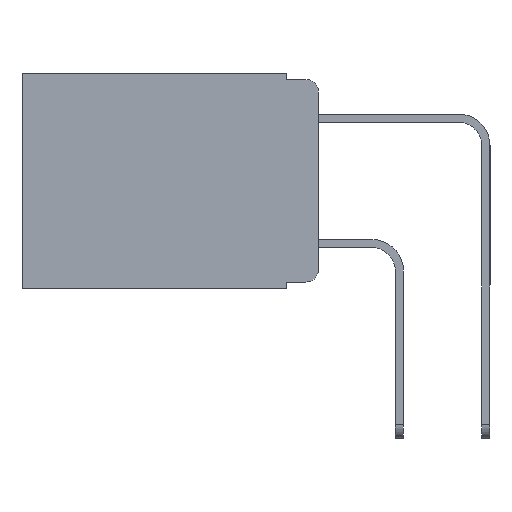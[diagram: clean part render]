
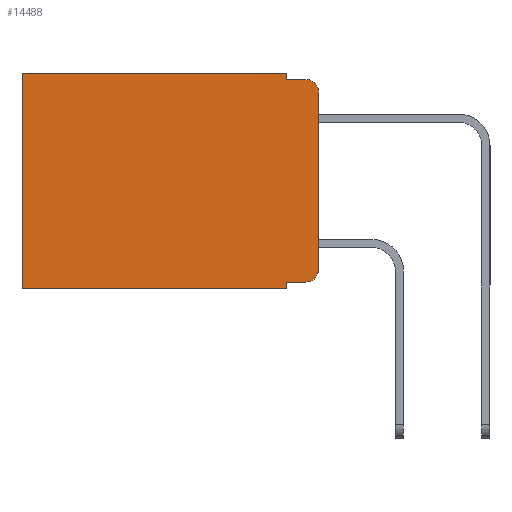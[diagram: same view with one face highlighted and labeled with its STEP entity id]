
A CAD part, left-side view. The second image highlights one B-rep face of the part: STEP entity #14488.
In plain terms, the highlighted planar face has unit normal (-1, 0, 0).
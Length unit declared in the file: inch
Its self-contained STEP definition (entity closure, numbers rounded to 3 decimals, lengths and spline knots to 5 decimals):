
#124 = LINE ( 'NONE', #17077, #3722 ) ;
#168 = CARTESIAN_POINT ( 'NONE',  ( 0.298, 0.02, -0.03 ) ) ;
#318 = VECTOR ( 'NONE', #9540, 39.37008 ) ;
#708 = EDGE_CURVE ( 'NONE', #4580, #9162, #13076, .T. ) ;
#1223 = DIRECTION ( 'NONE',  ( 0., 0., -1. ) ) ;
#1739 = DIRECTION ( 'NONE',  ( 0., 0., -1. ) ) ;
#1746 = EDGE_CURVE ( 'NONE', #9448, #4987, #8226, .T. ) ;
#2218 = CARTESIAN_POINT ( 'NONE',  ( 0.298, 0., 0. ) ) ;
#2753 = EDGE_CURVE ( 'NONE', #8319, #12787, #11417, .T. ) ;
#2843 = ORIENTED_EDGE ( 'NONE', *, *, #17005, .T. ) ;
#2996 = CARTESIAN_POINT ( 'NONE',  ( 0.298, 0.473, -0.343 ) ) ;
#3267 = EDGE_CURVE ( 'NONE', #8319, #9448, #16802, .T. ) ;
#3722 = VECTOR ( 'NONE', #14476, 39.37008 ) ;
#3731 = DIRECTION ( 'NONE',  ( 0., 1., 0. ) ) ;
#3923 = VECTOR ( 'NONE', #7118, 39.37008 ) ;
#3963 = CARTESIAN_POINT ( 'NONE',  ( 0.298, 0.051, 0. ) ) ;
#4008 = DIRECTION ( 'NONE',  ( 0., 0., -1. ) ) ;
#4037 = CARTESIAN_POINT ( 'NONE',  ( 0.298, 0.02, -0.01 ) ) ;
#4163 = DIRECTION ( 'NONE',  ( -1., 0., 0. ) ) ;
#4171 = DIRECTION ( 'NONE',  ( 0., 1., 0. ) ) ;
#4580 = VERTEX_POINT ( 'NONE', #17261 ) ;
#4729 = CIRCLE ( 'NONE', #5491, 0.02 ) ;
#4805 = EDGE_CURVE ( 'NONE', #12787, #11302, #15932, .T. ) ;
#4987 = VERTEX_POINT ( 'NONE', #2996 ) ;
#5491 = AXIS2_PLACEMENT_3D ( 'NONE', #12507, #4163, #13856 ) ;
#5778 = EDGE_CURVE ( 'NONE', #6436, #11302, #15610, .T. ) ;
#5812 = CARTESIAN_POINT ( 'NONE',  ( 0.298, 0.02, -0.333 ) ) ;
#6363 = DIRECTION ( 'NONE',  ( 1., 0., 0. ) ) ;
#6436 = VERTEX_POINT ( 'NONE', #11086 ) ;
#6603 = VERTEX_POINT ( 'NONE', #5812 ) ;
#6627 = ORIENTED_EDGE ( 'NONE', *, *, #13678, .F. ) ;
#7033 = ORIENTED_EDGE ( 'NONE', *, *, #2753, .F. ) ;
#7069 = CARTESIAN_POINT ( 'NONE',  ( 0.298, 0.051, -0.01 ) ) ;
#7118 = DIRECTION ( 'NONE',  ( 0., 0., -1. ) ) ;
#7306 = FACE_OUTER_BOUND ( 'NONE', #8794, .T. ) ;
#7647 = AXIS2_PLACEMENT_3D ( 'NONE', #7730, #6363, #15809 ) ;
#7717 = EDGE_CURVE ( 'NONE', #6436, #11690, #16570, .T. ) ;
#7730 = CARTESIAN_POINT ( 'NONE',  ( 0.298, 0., 0. ) ) ;
#7786 = CARTESIAN_POINT ( 'NONE',  ( 0.298, 0.051, 0. ) ) ;
#7909 = CARTESIAN_POINT ( 'NONE',  ( 0.298, 0.051, -0.01 ) ) ;
#8178 = CARTESIAN_POINT ( 'NONE',  ( 0.298, 0.473, 0. ) ) ;
#8226 = LINE ( 'NONE', #9786, #318 ) ;
#8319 = VERTEX_POINT ( 'NONE', #8489 ) ;
#8489 = CARTESIAN_POINT ( 'NONE',  ( 0.298, 0.051, 0. ) ) ;
#8794 = EDGE_LOOP ( 'NONE', ( #9149, #9576, #16069, #7033, #16908, #17750, #6627, #11867, #2843, #14637 ) ) ;
#9064 = VECTOR ( 'NONE', #1223, 39.37008 ) ;
#9149 = ORIENTED_EDGE ( 'NONE', *, *, #7717, .F. ) ;
#9162 = VERTEX_POINT ( 'NONE', #15621 ) ;
#9448 = VERTEX_POINT ( 'NONE', #8178 ) ;
#9540 = DIRECTION ( 'NONE',  ( 0., 0., -1. ) ) ;
#9576 = ORIENTED_EDGE ( 'NONE', *, *, #5778, .T. ) ;
#9786 = CARTESIAN_POINT ( 'NONE',  ( 0.298, 0.473, 0. ) ) ;
#9830 = DIRECTION ( 'NONE',  ( 0., -1., 0. ) ) ;
#10286 = AXIS2_PLACEMENT_3D ( 'NONE', #168, #10379, #1739 ) ;
#10379 = DIRECTION ( 'NONE',  ( -1., 0., 0. ) ) ;
#10656 = CARTESIAN_POINT ( 'NONE',  ( 0.298, 0., -0.313 ) ) ;
#10990 = VECTOR ( 'NONE', #3731, 39.37008 ) ;
#11086 = CARTESIAN_POINT ( 'NONE',  ( 0.298, 0., -0.03 ) ) ;
#11302 = VERTEX_POINT ( 'NONE', #4037 ) ;
#11417 = LINE ( 'NONE', #7786, #3923 ) ;
#11690 = VERTEX_POINT ( 'NONE', #10656 ) ;
#11867 = ORIENTED_EDGE ( 'NONE', *, *, #708, .F. ) ;
#12507 = CARTESIAN_POINT ( 'NONE',  ( 0.298, 0.02, -0.313 ) ) ;
#12787 = VERTEX_POINT ( 'NONE', #7909 ) ;
#13076 = LINE ( 'NONE', #3963, #16198 ) ;
#13678 = EDGE_CURVE ( 'NONE', #9162, #4987, #14490, .T. ) ;
#13856 = DIRECTION ( 'NONE',  ( 0., 0., -1. ) ) ;
#14073 = VECTOR ( 'NONE', #4171, 39.37008 ) ;
#14280 = VECTOR ( 'NONE', #9830, 39.37008 ) ;
#14476 = DIRECTION ( 'NONE',  ( 0., -1., 0. ) ) ;
#14486 = PLANE ( 'NONE',  #7647 ) ;
#14488 = ADVANCED_FACE ( 'NONE', ( #7306 ), #14486, .F. ) ;
#14490 = LINE ( 'NONE', #15275, #14073 ) ;
#14637 = ORIENTED_EDGE ( 'NONE', *, *, #16113, .T. ) ;
#15275 = CARTESIAN_POINT ( 'NONE',  ( 0.298, 0., -0.343 ) ) ;
#15610 = CIRCLE ( 'NONE', #10286, 0.02 ) ;
#15621 = CARTESIAN_POINT ( 'NONE',  ( 0.298, 0.051, -0.343 ) ) ;
#15809 = DIRECTION ( 'NONE',  ( 0., 0., -1. ) ) ;
#15932 = LINE ( 'NONE', #7069, #14280 ) ;
#16069 = ORIENTED_EDGE ( 'NONE', *, *, #4805, .F. ) ;
#16113 = EDGE_CURVE ( 'NONE', #6603, #11690, #4729, .T. ) ;
#16198 = VECTOR ( 'NONE', #4008, 39.37008 ) ;
#16570 = LINE ( 'NONE', #17971, #9064 ) ;
#16802 = LINE ( 'NONE', #2218, #10990 ) ;
#16908 = ORIENTED_EDGE ( 'NONE', *, *, #3267, .T. ) ;
#17005 = EDGE_CURVE ( 'NONE', #4580, #6603, #124, .T. ) ;
#17077 = CARTESIAN_POINT ( 'NONE',  ( 0.298, 0.051, -0.333 ) ) ;
#17261 = CARTESIAN_POINT ( 'NONE',  ( 0.298, 0.051, -0.333 ) ) ;
#17750 = ORIENTED_EDGE ( 'NONE', *, *, #1746, .T. ) ;
#17971 = CARTESIAN_POINT ( 'NONE',  ( 0.298, 0., 0. ) ) ;
